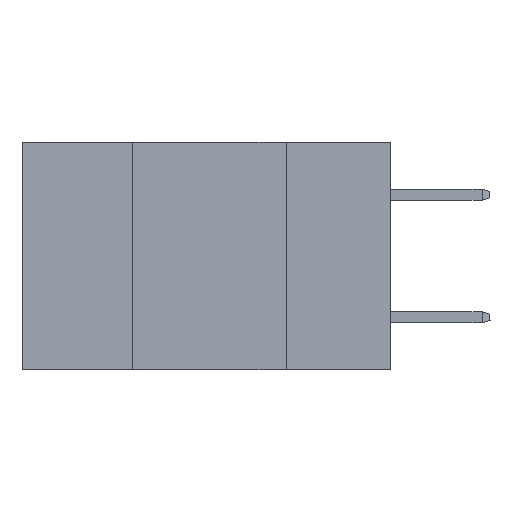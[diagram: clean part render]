
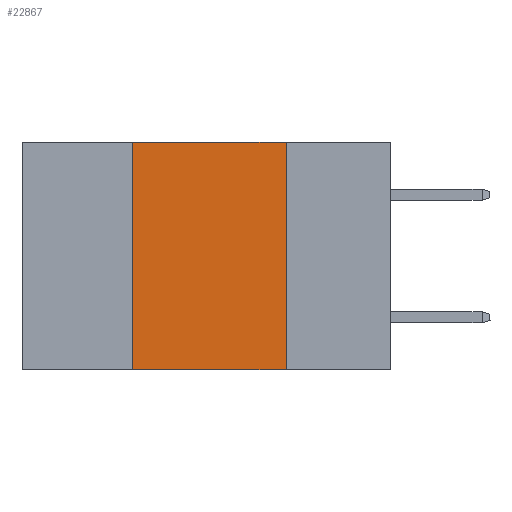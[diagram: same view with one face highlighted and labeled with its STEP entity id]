
A CAD part, left-side view. The second image highlights one B-rep face of the part: STEP entity #22867.
In plain terms, the highlighted planar face has unit normal (-1, 0, 0).
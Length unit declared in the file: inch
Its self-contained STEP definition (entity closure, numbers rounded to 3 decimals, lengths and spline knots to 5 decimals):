
#43 = ORIENTED_EDGE ( 'NONE', *, *, #38322, .F. ) ;
#1150 = CARTESIAN_POINT ( 'NONE',  ( 0., 0.6, 0. ) ) ;
#1969 = LINE ( 'NONE', #8722, #33649 ) ;
#2031 = EDGE_CURVE ( 'NONE', #8555, #18848, #39735, .T. ) ;
#3132 = CARTESIAN_POINT ( 'NONE',  ( 0., 0.6, -0.37 ) ) ;
#3529 = DIRECTION ( 'NONE',  ( 0., 0., -1. ) ) ;
#4144 = CARTESIAN_POINT ( 'NONE',  ( 0., 0.17, -0.37 ) ) ;
#5529 = AXIS2_PLACEMENT_3D ( 'NONE', #31686, #24243, #3529 ) ;
#8296 = ORIENTED_EDGE ( 'NONE', *, *, #45055, .F. ) ;
#8555 = VERTEX_POINT ( 'NONE', #29339 ) ;
#8722 = CARTESIAN_POINT ( 'NONE',  ( 0., 0.17, 0. ) ) ;
#12212 = EDGE_LOOP ( 'NONE', ( #8296, #26373, #43, #20848 ) ) ;
#14183 = CARTESIAN_POINT ( 'NONE',  ( 0., 0.42, 0. ) ) ;
#14867 = VERTEX_POINT ( 'NONE', #14183 ) ;
#15348 = VECTOR ( 'NONE', #31292, 39.37008 ) ;
#17489 = FACE_OUTER_BOUND ( 'NONE', #12212, .T. ) ;
#18363 = DIRECTION ( 'NONE',  ( 0., -1., 0. ) ) ;
#18440 = VERTEX_POINT ( 'NONE', #24684 ) ;
#18848 = VERTEX_POINT ( 'NONE', #4144 ) ;
#20848 = ORIENTED_EDGE ( 'NONE', *, *, #2031, .T. ) ;
#22174 = VECTOR ( 'NONE', #30158, 39.37008 ) ;
#22867 = ADVANCED_FACE ( 'NONE', ( #17489 ), #27966, .F. ) ;
#24243 = DIRECTION ( 'NONE',  ( 1., 0., 0. ) ) ;
#24684 = CARTESIAN_POINT ( 'NONE',  ( 0., 0.17, 0. ) ) ;
#24939 = VECTOR ( 'NONE', #18363, 39.37008 ) ;
#26373 = ORIENTED_EDGE ( 'NONE', *, *, #32633, .F. ) ;
#27370 = LINE ( 'NONE', #30620, #22174 ) ;
#27966 = PLANE ( 'NONE',  #5529 ) ;
#29339 = CARTESIAN_POINT ( 'NONE',  ( 0., 0.42, -0.37 ) ) ;
#30158 = DIRECTION ( 'NONE',  ( 0., 0., 1. ) ) ;
#30620 = CARTESIAN_POINT ( 'NONE',  ( 0., 0.42, 0. ) ) ;
#31292 = DIRECTION ( 'NONE',  ( 0., -1., 0. ) ) ;
#31686 = CARTESIAN_POINT ( 'NONE',  ( 0., 0.6, 0. ) ) ;
#32565 = LINE ( 'NONE', #1150, #24939 ) ;
#32633 = EDGE_CURVE ( 'NONE', #14867, #18440, #32565, .T. ) ;
#33649 = VECTOR ( 'NONE', #40595, 39.37008 ) ;
#38322 = EDGE_CURVE ( 'NONE', #8555, #14867, #27370, .T. ) ;
#39735 = LINE ( 'NONE', #3132, #15348 ) ;
#40595 = DIRECTION ( 'NONE',  ( 0., 0., -1. ) ) ;
#45055 = EDGE_CURVE ( 'NONE', #18440, #18848, #1969, .T. ) ;
